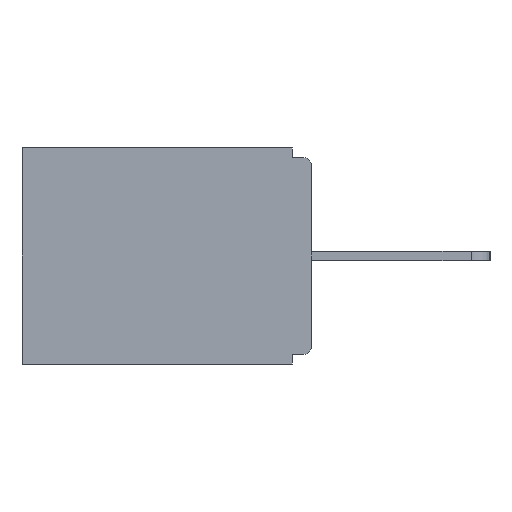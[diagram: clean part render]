
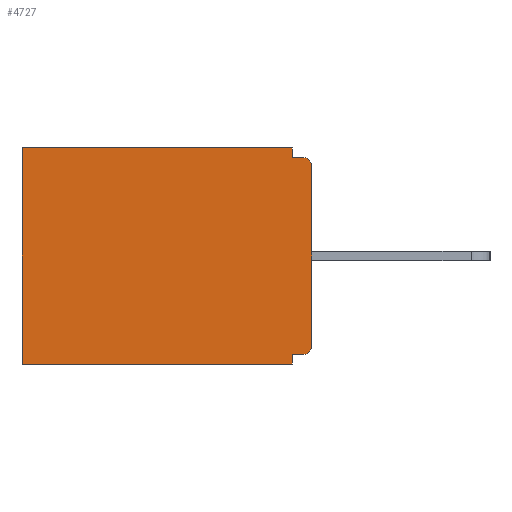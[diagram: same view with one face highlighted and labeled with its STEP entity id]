
A CAD part, left-side view. The second image highlights one B-rep face of the part: STEP entity #4727.
In plain terms, the highlighted planar face has unit normal (-1, 0, 0).
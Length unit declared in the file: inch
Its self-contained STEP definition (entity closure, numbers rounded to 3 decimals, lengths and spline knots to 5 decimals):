
#7 = ORIENTED_EDGE ( 'NONE', *, *, #15191, .F. ) ;
#120 = CARTESIAN_POINT ( 'NONE',  ( 0.298, 0., 0. ) ) ;
#627 = LINE ( 'NONE', #11519, #16501 ) ;
#675 = CARTESIAN_POINT ( 'NONE',  ( 0.298, 0.031, -0.328 ) ) ;
#758 = ORIENTED_EDGE ( 'NONE', *, *, #16855, .F. ) ;
#1289 = CARTESIAN_POINT ( 'NONE',  ( 0.298, 0., -0.03 ) ) ;
#1316 = ORIENTED_EDGE ( 'NONE', *, *, #11447, .F. ) ;
#1349 = ORIENTED_EDGE ( 'NONE', *, *, #15644, .T. ) ;
#1379 = VERTEX_POINT ( 'NONE', #13059 ) ;
#1465 = ORIENTED_EDGE ( 'NONE', *, *, #16132, .F. ) ;
#1466 = EDGE_CURVE ( 'NONE', #5580, #16547, #18123, .T. ) ;
#1653 = AXIS2_PLACEMENT_3D ( 'NONE', #15050, #5875, #16537 ) ;
#1664 = DIRECTION ( 'NONE',  ( 0., 0., -1. ) ) ;
#1903 = CARTESIAN_POINT ( 'NONE',  ( 0.298, 0.031, -0.015 ) ) ;
#2212 = CARTESIAN_POINT ( 'NONE',  ( 0.298, 0.015, -0.015 ) ) ;
#3256 = VERTEX_POINT ( 'NONE', #1903 ) ;
#3527 = DIRECTION ( 'NONE',  ( 0., 0., -1. ) ) ;
#3622 = EDGE_CURVE ( 'NONE', #3256, #16490, #8397, .T. ) ;
#4568 = ORIENTED_EDGE ( 'NONE', *, *, #7551, .T. ) ;
#4587 = LINE ( 'NONE', #8820, #11421 ) ;
#4727 = ADVANCED_FACE ( 'NONE', ( #7625 ), #5576, .F. ) ;
#5330 = DIRECTION ( 'NONE',  ( 0., 0., -1. ) ) ;
#5576 = PLANE ( 'NONE',  #10313 ) ;
#5580 = VERTEX_POINT ( 'NONE', #12188 ) ;
#5714 = VERTEX_POINT ( 'NONE', #16668 ) ;
#5875 = DIRECTION ( 'NONE',  ( -1., 0., 0. ) ) ;
#6343 = CARTESIAN_POINT ( 'NONE',  ( 0.298, 0.015, -0.03 ) ) ;
#6354 = VERTEX_POINT ( 'NONE', #675 ) ;
#6478 = ORIENTED_EDGE ( 'NONE', *, *, #1466, .T. ) ;
#6587 = ORIENTED_EDGE ( 'NONE', *, *, #18005, .T. ) ;
#6736 = VERTEX_POINT ( 'NONE', #17759 ) ;
#6753 = VERTEX_POINT ( 'NONE', #8016 ) ;
#7463 = VECTOR ( 'NONE', #14048, 39.37008 ) ;
#7551 = EDGE_CURVE ( 'NONE', #9044, #16490, #18699, .T. ) ;
#7625 = FACE_OUTER_BOUND ( 'NONE', #13882, .T. ) ;
#8016 = CARTESIAN_POINT ( 'NONE',  ( 0.298, 0., -0.313 ) ) ;
#8040 = DIRECTION ( 'NONE',  ( 1., 0., 0. ) ) ;
#8067 = DIRECTION ( 'NONE',  ( 0., -1., 0. ) ) ;
#8397 = LINE ( 'NONE', #17486, #16452 ) ;
#8434 = DIRECTION ( 'NONE',  ( -1., 0., 0. ) ) ;
#8442 = DIRECTION ( 'NONE',  ( 0., 0., -1. ) ) ;
#8764 = ORIENTED_EDGE ( 'NONE', *, *, #3622, .F. ) ;
#8820 = CARTESIAN_POINT ( 'NONE',  ( 0.298, 0., -0.343 ) ) ;
#8867 = VECTOR ( 'NONE', #12557, 39.37008 ) ;
#9044 = VERTEX_POINT ( 'NONE', #1289 ) ;
#9109 = CARTESIAN_POINT ( 'NONE',  ( 0.298, 0., -0.328 ) ) ;
#9259 = CARTESIAN_POINT ( 'NONE',  ( 0.298, 0., 0. ) ) ;
#9361 = LINE ( 'NONE', #120, #8867 ) ;
#9827 = LINE ( 'NONE', #15525, #13403 ) ;
#10313 = AXIS2_PLACEMENT_3D ( 'NONE', #9259, #8040, #3527 ) ;
#10398 = DIRECTION ( 'NONE',  ( 0., 1., 0. ) ) ;
#10622 = LINE ( 'NONE', #9109, #15069 ) ;
#10689 = DIRECTION ( 'NONE',  ( 0., 1., 0. ) ) ;
#11421 = VECTOR ( 'NONE', #10398, 39.37008 ) ;
#11447 = EDGE_CURVE ( 'NONE', #6354, #1379, #9827, .T. ) ;
#11519 = CARTESIAN_POINT ( 'NONE',  ( 0.298, 0.031, -0.343 ) ) ;
#11705 = CARTESIAN_POINT ( 'NONE',  ( 0.298, 0.46, -0.343 ) ) ;
#12188 = CARTESIAN_POINT ( 'NONE',  ( 0.298, 0.46, 0. ) ) ;
#12539 = CARTESIAN_POINT ( 'NONE',  ( 0.298, 0., 0. ) ) ;
#12557 = DIRECTION ( 'NONE',  ( 0., 0., -1. ) ) ;
#13015 = CARTESIAN_POINT ( 'NONE',  ( 0.298, 0.46, 0. ) ) ;
#13059 = CARTESIAN_POINT ( 'NONE',  ( 0.298, 0.031, -0.343 ) ) ;
#13403 = VECTOR ( 'NONE', #1664, 39.37008 ) ;
#13882 = EDGE_LOOP ( 'NONE', ( #4568, #8764, #7, #1349, #6478, #14859, #1316, #1465, #6587, #758 ) ) ;
#14048 = DIRECTION ( 'NONE',  ( 0., 1., 0. ) ) ;
#14859 = ORIENTED_EDGE ( 'NONE', *, *, #19687, .F. ) ;
#15050 = CARTESIAN_POINT ( 'NONE',  ( 0.298, 0.015, -0.313 ) ) ;
#15069 = VECTOR ( 'NONE', #10689, 39.37008 ) ;
#15191 = EDGE_CURVE ( 'NONE', #6736, #3256, #627, .T. ) ;
#15525 = CARTESIAN_POINT ( 'NONE',  ( 0.298, 0.031, -0.343 ) ) ;
#15644 = EDGE_CURVE ( 'NONE', #6736, #5580, #19452, .T. ) ;
#16109 = DIRECTION ( 'NONE',  ( 0., 0., -1. ) ) ;
#16132 = EDGE_CURVE ( 'NONE', #5714, #6354, #10622, .T. ) ;
#16452 = VECTOR ( 'NONE', #8067, 39.37008 ) ;
#16490 = VERTEX_POINT ( 'NONE', #2212 ) ;
#16501 = VECTOR ( 'NONE', #5330, 39.37008 ) ;
#16537 = DIRECTION ( 'NONE',  ( 0., 0., -1. ) ) ;
#16547 = VERTEX_POINT ( 'NONE', #11705 ) ;
#16668 = CARTESIAN_POINT ( 'NONE',  ( 0.298, 0.015, -0.328 ) ) ;
#16855 = EDGE_CURVE ( 'NONE', #9044, #6753, #9361, .T. ) ;
#17217 = AXIS2_PLACEMENT_3D ( 'NONE', #6343, #8434, #8442 ) ;
#17486 = CARTESIAN_POINT ( 'NONE',  ( 0.298, 0., -0.015 ) ) ;
#17681 = VECTOR ( 'NONE', #16109, 39.37008 ) ;
#17759 = CARTESIAN_POINT ( 'NONE',  ( 0.298, 0.031, 0. ) ) ;
#18005 = EDGE_CURVE ( 'NONE', #5714, #6753, #19593, .T. ) ;
#18123 = LINE ( 'NONE', #13015, #17681 ) ;
#18699 = CIRCLE ( 'NONE', #17217, 0.015 ) ;
#19452 = LINE ( 'NONE', #12539, #7463 ) ;
#19593 = CIRCLE ( 'NONE', #1653, 0.015 ) ;
#19687 = EDGE_CURVE ( 'NONE', #1379, #16547, #4587, .T. ) ;
